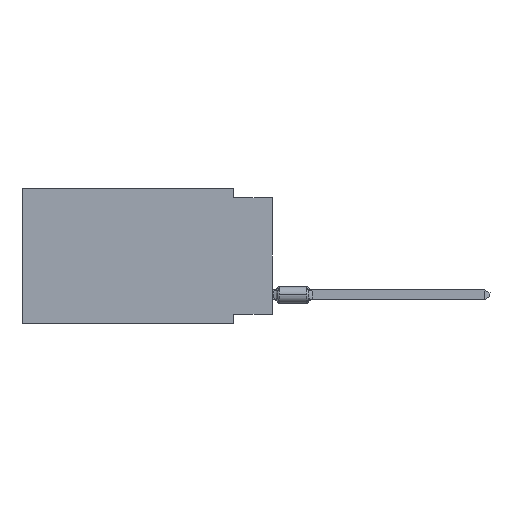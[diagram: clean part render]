
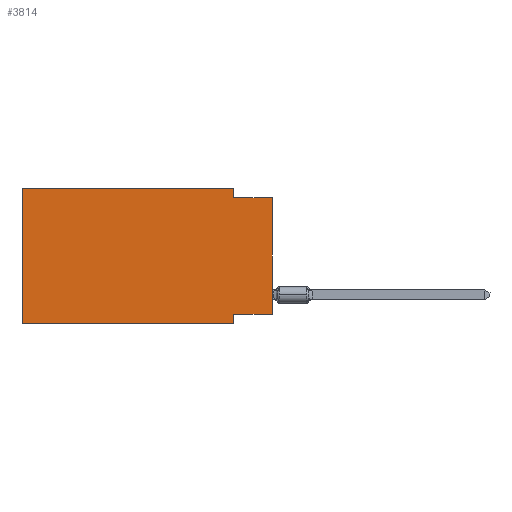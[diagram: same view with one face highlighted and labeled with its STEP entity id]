
A CAD part, left-side view. The second image highlights one B-rep face of the part: STEP entity #3814.
In plain terms, the highlighted planar face has unit normal (-1, 0, 0).
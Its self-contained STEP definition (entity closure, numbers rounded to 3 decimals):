
#213 = VECTOR ( 'NONE', #6237, 1000. ) ;
#229 = VECTOR ( 'NONE', #5411, 1000. ) ;
#590 = LINE ( 'NONE', #3911, #6681 ) ;
#626 = DIRECTION ( 'NONE',  ( 1., 0., 0. ) ) ;
#667 = DIRECTION ( 'NONE',  ( 0., 1., 0. ) ) ;
#1661 = LINE ( 'NONE', #13283, #213 ) ;
#1687 = CARTESIAN_POINT ( 'NONE',  ( 0., 16.383, 0. ) ) ;
#1769 = PLANE ( 'NONE',  #7236 ) ;
#1903 = VECTOR ( 'NONE', #667, 1000. ) ;
#2614 = CARTESIAN_POINT ( 'NONE',  ( 0., 0., 0. ) ) ;
#2727 = CARTESIAN_POINT ( 'NONE',  ( 0., 16.383, 0. ) ) ;
#2773 = LINE ( 'NONE', #9898, #1903 ) ;
#2829 = CARTESIAN_POINT ( 'NONE',  ( 0., 2.54, -8.255 ) ) ;
#2852 = VECTOR ( 'NONE', #7086, 1000. ) ;
#2901 = ORIENTED_EDGE ( 'NONE', *, *, #12738, .F. ) ;
#2905 = VERTEX_POINT ( 'NONE', #14117 ) ;
#2923 = DIRECTION ( 'NONE',  ( 0., -1., 0. ) ) ;
#3154 = CARTESIAN_POINT ( 'NONE',  ( 0., 2.54, -0.635 ) ) ;
#3519 = CARTESIAN_POINT ( 'NONE',  ( 0., 0., -8.255 ) ) ;
#3669 = LINE ( 'NONE', #8230, #4027 ) ;
#3749 = LINE ( 'NONE', #2614, #5495 ) ;
#3814 = ADVANCED_FACE ( 'NONE', ( #12055 ), #1769, .F. ) ;
#3911 = CARTESIAN_POINT ( 'NONE',  ( 0., 0., -0.635 ) ) ;
#3953 = ORIENTED_EDGE ( 'NONE', *, *, #13460, .T. ) ;
#4027 = VECTOR ( 'NONE', #10563, 1000. ) ;
#5172 = EDGE_CURVE ( 'NONE', #12505, #8060, #9252, .T. ) ;
#5411 = DIRECTION ( 'NONE',  ( 0., -1., 0. ) ) ;
#5495 = VECTOR ( 'NONE', #10423, 1000. ) ;
#5515 = EDGE_CURVE ( 'NONE', #12279, #13543, #590, .T. ) ;
#6237 = DIRECTION ( 'NONE',  ( 0., -1., 0. ) ) ;
#6681 = VECTOR ( 'NONE', #2923, 1000. ) ;
#6882 = CARTESIAN_POINT ( 'NONE',  ( 0., 2.54, -8.89 ) ) ;
#6995 = ORIENTED_EDGE ( 'NONE', *, *, #5515, .F. ) ;
#7086 = DIRECTION ( 'NONE',  ( 0., 0., -1. ) ) ;
#7142 = EDGE_LOOP ( 'NONE', ( #3953, #6995, #12860, #7285, #2901, #14359, #12887, #8942 ) ) ;
#7236 = AXIS2_PLACEMENT_3D ( 'NONE', #13099, #626, #9995 ) ;
#7285 = ORIENTED_EDGE ( 'NONE', *, *, #11672, .F. ) ;
#8060 = VERTEX_POINT ( 'NONE', #6882 ) ;
#8183 = VERTEX_POINT ( 'NONE', #3519 ) ;
#8230 = CARTESIAN_POINT ( 'NONE',  ( 0., 16.383, 0. ) ) ;
#8942 = ORIENTED_EDGE ( 'NONE', *, *, #12157, .F. ) ;
#9187 = CARTESIAN_POINT ( 'NONE',  ( 0., 2.54, -8.89 ) ) ;
#9252 = LINE ( 'NONE', #9187, #2852 ) ;
#9866 = CARTESIAN_POINT ( 'NONE',  ( 0., 0., -0.635 ) ) ;
#9898 = CARTESIAN_POINT ( 'NONE',  ( 0., 0., -8.255 ) ) ;
#9995 = DIRECTION ( 'NONE',  ( 0., 0., -1. ) ) ;
#10423 = DIRECTION ( 'NONE',  ( 0., 0., 1. ) ) ;
#10509 = VECTOR ( 'NONE', #14481, 1000. ) ;
#10563 = DIRECTION ( 'NONE',  ( 0., 0., 1. ) ) ;
#11051 = CARTESIAN_POINT ( 'NONE',  ( 0., 2.54, 0. ) ) ;
#11628 = VERTEX_POINT ( 'NONE', #2727 ) ;
#11672 = EDGE_CURVE ( 'NONE', #11628, #11737, #12257, .T. ) ;
#11737 = VERTEX_POINT ( 'NONE', #11051 ) ;
#12055 = FACE_OUTER_BOUND ( 'NONE', #7142, .T. ) ;
#12157 = EDGE_CURVE ( 'NONE', #8183, #12505, #2773, .T. ) ;
#12237 = CARTESIAN_POINT ( 'NONE',  ( 0., 2.54, 0. ) ) ;
#12257 = LINE ( 'NONE', #1687, #229 ) ;
#12279 = VERTEX_POINT ( 'NONE', #3154 ) ;
#12505 = VERTEX_POINT ( 'NONE', #2829 ) ;
#12738 = EDGE_CURVE ( 'NONE', #2905, #11628, #3669, .T. ) ;
#12860 = ORIENTED_EDGE ( 'NONE', *, *, #13119, .F. ) ;
#12887 = ORIENTED_EDGE ( 'NONE', *, *, #5172, .F. ) ;
#13099 = CARTESIAN_POINT ( 'NONE',  ( 0., 16.383, 0. ) ) ;
#13115 = EDGE_CURVE ( 'NONE', #2905, #8060, #1661, .T. ) ;
#13119 = EDGE_CURVE ( 'NONE', #11737, #12279, #14416, .T. ) ;
#13283 = CARTESIAN_POINT ( 'NONE',  ( 0., 16.383, -8.89 ) ) ;
#13460 = EDGE_CURVE ( 'NONE', #8183, #13543, #3749, .T. ) ;
#13543 = VERTEX_POINT ( 'NONE', #9866 ) ;
#14117 = CARTESIAN_POINT ( 'NONE',  ( 0., 16.383, -8.89 ) ) ;
#14359 = ORIENTED_EDGE ( 'NONE', *, *, #13115, .T. ) ;
#14416 = LINE ( 'NONE', #12237, #10509 ) ;
#14481 = DIRECTION ( 'NONE',  ( 0., 0., -1. ) ) ;
